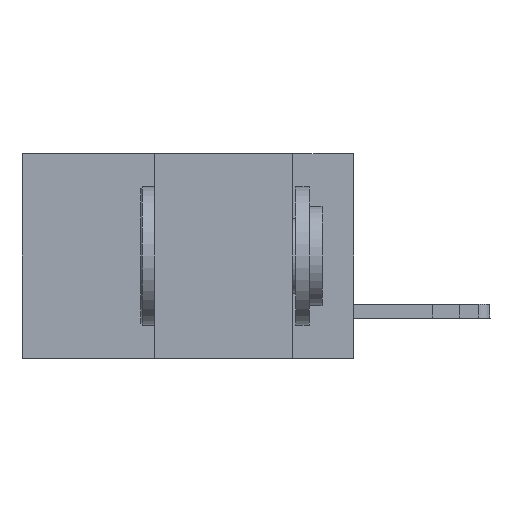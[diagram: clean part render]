
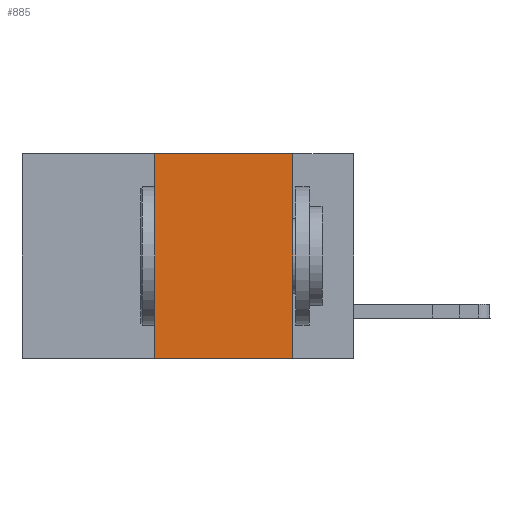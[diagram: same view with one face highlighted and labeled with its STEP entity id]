
A CAD part, left-side view. The second image highlights one B-rep face of the part: STEP entity #885.
In plain terms, the highlighted planar face has unit normal (-1, 0, 0).
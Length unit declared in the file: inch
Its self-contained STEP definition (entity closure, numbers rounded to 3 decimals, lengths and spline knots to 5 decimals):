
#166 = VECTOR ( 'NONE', #11268, 39.37008 ) ;
#195 = VERTEX_POINT ( 'NONE', #5861 ) ;
#330 = ORIENTED_EDGE ( 'NONE', *, *, #9231, .F. ) ;
#885 = ADVANCED_FACE ( 'NONE', ( #16854 ), #14110, .F. ) ;
#1983 = ORIENTED_EDGE ( 'NONE', *, *, #15615, .F. ) ;
#2141 = VECTOR ( 'NONE', #5660, 39.37008 ) ;
#3156 = LINE ( 'NONE', #7481, #10613 ) ;
#4935 = EDGE_CURVE ( 'NONE', #195, #6210, #6080, .T. ) ;
#5340 = CARTESIAN_POINT ( 'NONE',  ( 0., 0.11, 0. ) ) ;
#5660 = DIRECTION ( 'NONE',  ( 0., -1., 0. ) ) ;
#5861 = CARTESIAN_POINT ( 'NONE',  ( 0., 0.36, 0. ) ) ;
#5956 = DIRECTION ( 'NONE',  ( 0., -1., 0. ) ) ;
#6080 = LINE ( 'NONE', #11613, #2141 ) ;
#6210 = VERTEX_POINT ( 'NONE', #16207 ) ;
#7481 = CARTESIAN_POINT ( 'NONE',  ( 0., 0.36, 0. ) ) ;
#8290 = ORIENTED_EDGE ( 'NONE', *, *, #17327, .T. ) ;
#9224 = CARTESIAN_POINT ( 'NONE',  ( 0., 0.36, -0.37 ) ) ;
#9231 = EDGE_CURVE ( 'NONE', #13583, #195, #3156, .T. ) ;
#9897 = ORIENTED_EDGE ( 'NONE', *, *, #4935, .F. ) ;
#10377 = CARTESIAN_POINT ( 'NONE',  ( 0., 0.6, 0. ) ) ;
#10613 = VECTOR ( 'NONE', #17939, 39.37008 ) ;
#11268 = DIRECTION ( 'NONE',  ( 0., 0., -1. ) ) ;
#11478 = DIRECTION ( 'NONE',  ( 0., 0., -1. ) ) ;
#11613 = CARTESIAN_POINT ( 'NONE',  ( 0., 0.6, 0. ) ) ;
#11696 = VERTEX_POINT ( 'NONE', #13252 ) ;
#12556 = EDGE_LOOP ( 'NONE', ( #1983, #9897, #330, #8290 ) ) ;
#13252 = CARTESIAN_POINT ( 'NONE',  ( 0., 0.11, -0.37 ) ) ;
#13408 = CARTESIAN_POINT ( 'NONE',  ( 0., 0.6, -0.37 ) ) ;
#13583 = VERTEX_POINT ( 'NONE', #9224 ) ;
#14110 = PLANE ( 'NONE',  #17288 ) ;
#15333 = LINE ( 'NONE', #13408, #19279 ) ;
#15615 = EDGE_CURVE ( 'NONE', #6210, #11696, #16056, .T. ) ;
#16056 = LINE ( 'NONE', #5340, #166 ) ;
#16207 = CARTESIAN_POINT ( 'NONE',  ( 0., 0.11, 0. ) ) ;
#16854 = FACE_OUTER_BOUND ( 'NONE', #12556, .T. ) ;
#17288 = AXIS2_PLACEMENT_3D ( 'NONE', #10377, #17891, #11478 ) ;
#17327 = EDGE_CURVE ( 'NONE', #13583, #11696, #15333, .T. ) ;
#17891 = DIRECTION ( 'NONE',  ( 1., 0., 0. ) ) ;
#17939 = DIRECTION ( 'NONE',  ( 0., 0., 1. ) ) ;
#19279 = VECTOR ( 'NONE', #5956, 39.37008 ) ;
